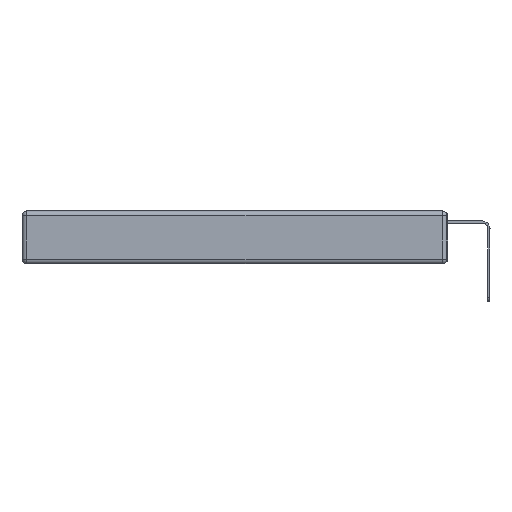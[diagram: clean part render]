
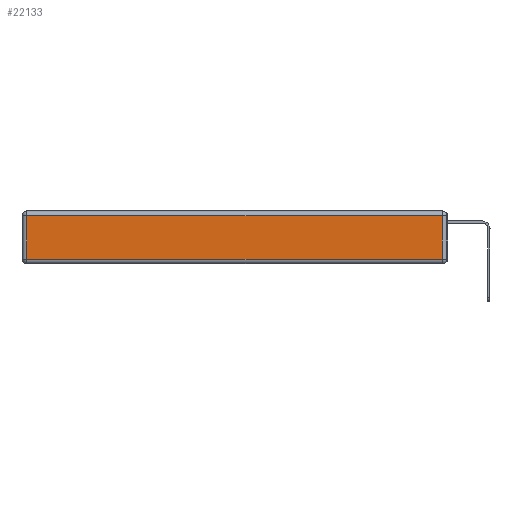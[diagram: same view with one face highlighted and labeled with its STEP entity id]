
A CAD part, left-side view. The second image highlights one B-rep face of the part: STEP entity #22133.
In plain terms, the highlighted planar face has unit normal (-1, 0, 0).
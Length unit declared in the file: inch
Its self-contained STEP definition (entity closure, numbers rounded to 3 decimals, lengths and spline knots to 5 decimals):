
#369 = ORIENTED_EDGE ( 'NONE', *, *, #18905, .T. ) ;
#1586 = CARTESIAN_POINT ( 'NONE',  ( 0., 2.72, -0.03 ) ) ;
#1832 = DIRECTION ( 'NONE',  ( 0., 0., 1. ) ) ;
#2001 = LINE ( 'NONE', #15021, #12154 ) ;
#2266 = AXIS2_PLACEMENT_3D ( 'NONE', #12307, #5727, #16397 ) ;
#3153 = EDGE_CURVE ( 'NONE', #16238, #16422, #2001, .T. ) ;
#3263 = VERTEX_POINT ( 'NONE', #11041 ) ;
#4233 = VERTEX_POINT ( 'NONE', #26124 ) ;
#4297 = CARTESIAN_POINT ( 'NONE',  ( 0., 2.72, -0.313 ) ) ;
#5310 = CARTESIAN_POINT ( 'NONE',  ( 0., 2.75, -0.03 ) ) ;
#5594 = DIRECTION ( 'NONE',  ( 0., 1., 0. ) ) ;
#5727 = DIRECTION ( 'NONE',  ( -1., 0., 0. ) ) ;
#6071 = ORIENTED_EDGE ( 'NONE', *, *, #9881, .T. ) ;
#6722 = ORIENTED_EDGE ( 'NONE', *, *, #12956, .T. ) ;
#7702 = VECTOR ( 'NONE', #27186, 39.37008 ) ;
#9881 = EDGE_CURVE ( 'NONE', #16422, #3263, #13506, .T. ) ;
#9925 = CARTESIAN_POINT ( 'NONE',  ( 0., 0., -0.313 ) ) ;
#10611 = CARTESIAN_POINT ( 'NONE',  ( 0., 0.03, -0.343 ) ) ;
#11041 = CARTESIAN_POINT ( 'NONE',  ( 0., 0.03, -0.313 ) ) ;
#12154 = VECTOR ( 'NONE', #23422, 39.37008 ) ;
#12307 = CARTESIAN_POINT ( 'NONE',  ( 0., 0., -0.343 ) ) ;
#12956 = EDGE_CURVE ( 'NONE', #3263, #4233, #21615, .T. ) ;
#13506 = LINE ( 'NONE', #9925, #7702 ) ;
#14862 = LINE ( 'NONE', #5310, #16481 ) ;
#15021 = CARTESIAN_POINT ( 'NONE',  ( 0., 2.72, -0.343 ) ) ;
#16238 = VERTEX_POINT ( 'NONE', #1586 ) ;
#16397 = DIRECTION ( 'NONE',  ( 0., 0., 1. ) ) ;
#16422 = VERTEX_POINT ( 'NONE', #4297 ) ;
#16481 = VECTOR ( 'NONE', #5594, 39.37008 ) ;
#17256 = VECTOR ( 'NONE', #1832, 39.37008 ) ;
#17425 = ORIENTED_EDGE ( 'NONE', *, *, #3153, .T. ) ;
#18448 = PLANE ( 'NONE',  #2266 ) ;
#18905 = EDGE_CURVE ( 'NONE', #4233, #16238, #14862, .T. ) ;
#21615 = LINE ( 'NONE', #10611, #17256 ) ;
#22133 = ADVANCED_FACE ( 'NONE', ( #22711 ), #18448, .T. ) ;
#22711 = FACE_OUTER_BOUND ( 'NONE', #26449, .T. ) ;
#23422 = DIRECTION ( 'NONE',  ( 0., 0., -1. ) ) ;
#26124 = CARTESIAN_POINT ( 'NONE',  ( 0., 0.03, -0.03 ) ) ;
#26449 = EDGE_LOOP ( 'NONE', ( #6071, #6722, #369, #17425 ) ) ;
#27186 = DIRECTION ( 'NONE',  ( 0., -1., 0. ) ) ;
